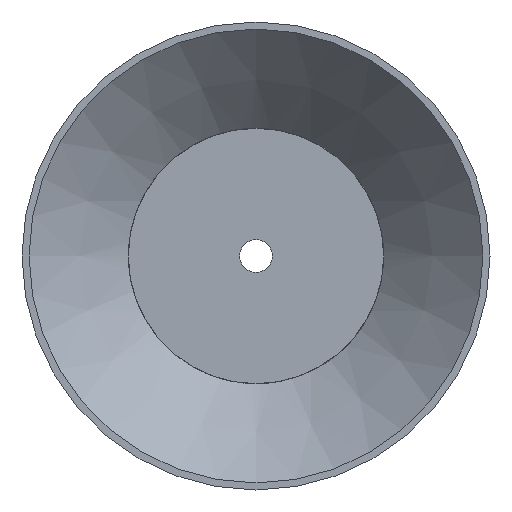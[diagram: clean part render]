
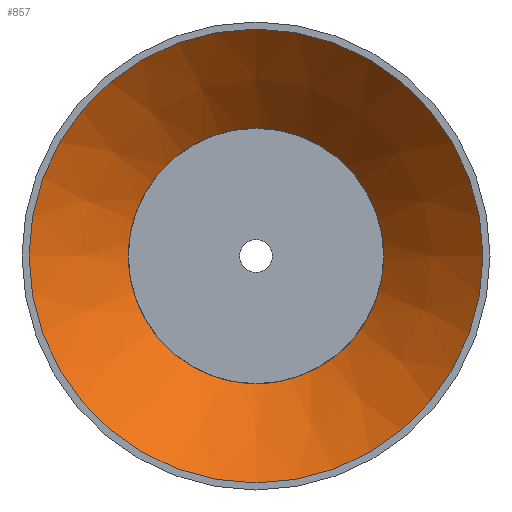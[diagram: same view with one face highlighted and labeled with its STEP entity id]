
A CAD part, front view. The second image highlights one B-rep face of the part: STEP entity #857.
In plain terms, the highlighted conical face has half-angle 45.227 degrees and reference radius 31.679 mm.
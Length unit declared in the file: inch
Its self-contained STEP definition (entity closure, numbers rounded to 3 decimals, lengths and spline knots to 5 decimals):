
#45=CONICAL_SURFACE('',#924,1.24722,0.789);
#54=LINE('',#1304,#84);
#84=VECTOR('',#1017,1.24722);
#116=(
BOUNDED_CURVE()
B_SPLINE_CURVE(2,(#1307,#1308,#1309),.UNSPECIFIED.,.F.,.F.)
B_SPLINE_CURVE_WITH_KNOTS((3,3),(0.,0.0225),.UNSPECIFIED.)
CURVE()
GEOMETRIC_REPRESENTATION_ITEM()
RATIONAL_B_SPLINE_CURVE((1.,1.,1.))
REPRESENTATION_ITEM('')
);
#117=(
BOUNDED_CURVE()
B_SPLINE_CURVE(2,(#1311,#1312,#1313),.UNSPECIFIED.,.F.,.F.)
B_SPLINE_CURVE_WITH_KNOTS((3,3),(0.8627,0.8852),
 .UNSPECIFIED.)
CURVE()
GEOMETRIC_REPRESENTATION_ITEM()
RATIONAL_B_SPLINE_CURVE((1.,1.,1.))
REPRESENTATION_ITEM('')
);
#118=(
BOUNDED_CURVE()
B_SPLINE_CURVE(2,(#1316,#1317,#1318),.UNSPECIFIED.,.F.,.F.)
B_SPLINE_CURVE_WITH_KNOTS((3,3),(0.,0.0225),.UNSPECIFIED.)
CURVE()
GEOMETRIC_REPRESENTATION_ITEM()
RATIONAL_B_SPLINE_CURVE((1.,1.,1.))
REPRESENTATION_ITEM('')
);
#119=(
BOUNDED_CURVE()
B_SPLINE_CURVE(2,(#1320,#1321,#1322),.UNSPECIFIED.,.F.,.F.)
B_SPLINE_CURVE_WITH_KNOTS((3,3),(0.86268,0.88518),
 .UNSPECIFIED.)
CURVE()
GEOMETRIC_REPRESENTATION_ITEM()
RATIONAL_B_SPLINE_CURVE((1.,1.,1.))
REPRESENTATION_ITEM('')
);
#120=(
BOUNDED_CURVE()
B_SPLINE_CURVE(2,(#1325,#1326,#1327),.UNSPECIFIED.,.F.,.F.)
B_SPLINE_CURVE_WITH_KNOTS((3,3),(0.,0.0225),.UNSPECIFIED.)
CURVE()
GEOMETRIC_REPRESENTATION_ITEM()
RATIONAL_B_SPLINE_CURVE((1.,1.,1.))
REPRESENTATION_ITEM('')
);
#121=(
BOUNDED_CURVE()
B_SPLINE_CURVE(2,(#1329,#1330,#1331),.UNSPECIFIED.,.F.,.F.)
B_SPLINE_CURVE_WITH_KNOTS((3,3),(0.86263,0.88513),
 .UNSPECIFIED.)
CURVE()
GEOMETRIC_REPRESENTATION_ITEM()
RATIONAL_B_SPLINE_CURVE((1.,1.,1.))
REPRESENTATION_ITEM('')
);
#122=(
BOUNDED_CURVE()
B_SPLINE_CURVE(2,(#1335,#1336,#1337),.UNSPECIFIED.,.F.,.F.)
B_SPLINE_CURVE_WITH_KNOTS((3,3),(0.,0.0225),.UNSPECIFIED.)
CURVE()
GEOMETRIC_REPRESENTATION_ITEM()
RATIONAL_B_SPLINE_CURVE((1.,1.,1.))
REPRESENTATION_ITEM('')
);
#123=(
BOUNDED_CURVE()
B_SPLINE_CURVE(2,(#1341,#1342,#1343),.UNSPECIFIED.,.F.,.F.)
B_SPLINE_CURVE_WITH_KNOTS((3,3),(0.86258,0.88508),
 .UNSPECIFIED.)
CURVE()
GEOMETRIC_REPRESENTATION_ITEM()
RATIONAL_B_SPLINE_CURVE((1.,1.,1.))
REPRESENTATION_ITEM('')
);
#203=FACE_OUTER_BOUND('',#243,.T.);
#243=EDGE_LOOP('',(#606,#607,#608,#609,#610,#611,#612,#613,#614,#615,#616,
#617,#618,#619,#620,#621,#622,#623,#624,#625,#626));
#291=CIRCLE('',#919,0.89444);
#292=CIRCLE('',#921,0.89444);
#293=CIRCLE('',#923,0.89444);
#294=CIRCLE('',#925,1.6);
#295=CIRCLE('',#926,0.9);
#296=CIRCLE('',#927,0.9);
#297=CIRCLE('',#928,0.9);
#298=CIRCLE('',#929,0.9);
#299=CIRCLE('',#930,0.89444);
#300=CIRCLE('',#931,0.9);
#301=CIRCLE('',#932,1.6);
#338=VERTEX_POINT('',#1282);
#339=VERTEX_POINT('',#1284);
#340=VERTEX_POINT('',#1288);
#341=VERTEX_POINT('',#1290);
#342=VERTEX_POINT('',#1294);
#343=VERTEX_POINT('',#1296);
#344=VERTEX_POINT('',#1300);
#345=VERTEX_POINT('',#1301);
#346=VERTEX_POINT('',#1303);
#347=VERTEX_POINT('',#1305);
#348=VERTEX_POINT('',#1310);
#349=VERTEX_POINT('',#1314);
#350=VERTEX_POINT('',#1319);
#351=VERTEX_POINT('',#1323);
#352=VERTEX_POINT('',#1328);
#353=VERTEX_POINT('',#1332);
#354=VERTEX_POINT('',#1334);
#355=VERTEX_POINT('',#1338);
#356=VERTEX_POINT('',#1340);
#443=EDGE_CURVE('',#339,#338,#291,.T.);
#446=EDGE_CURVE('',#341,#340,#292,.T.);
#448=EDGE_CURVE('',#342,#343,#293,.T.);
#450=EDGE_CURVE('',#344,#345,#294,.T.);
#451=EDGE_CURVE('',#345,#346,#54,.T.);
#452=EDGE_CURVE('',#347,#346,#295,.T.);
#453=EDGE_CURVE('',#340,#347,#116,.T.);
#454=EDGE_CURVE('',#348,#341,#117,.T.);
#455=EDGE_CURVE('',#349,#348,#296,.T.);
#456=EDGE_CURVE('',#338,#349,#118,.T.);
#457=EDGE_CURVE('',#350,#339,#119,.T.);
#458=EDGE_CURVE('',#351,#350,#297,.T.);
#459=EDGE_CURVE('',#343,#351,#120,.T.);
#460=EDGE_CURVE('',#352,#342,#121,.T.);
#461=EDGE_CURVE('',#353,#352,#298,.T.);
#462=EDGE_CURVE('',#354,#353,#122,.T.);
#463=EDGE_CURVE('',#355,#354,#299,.T.);
#464=EDGE_CURVE('',#356,#355,#123,.T.);
#465=EDGE_CURVE('',#346,#356,#300,.T.);
#466=EDGE_CURVE('',#345,#344,#301,.T.);
#606=ORIENTED_EDGE('',*,*,#450,.T.);
#607=ORIENTED_EDGE('',*,*,#451,.T.);
#608=ORIENTED_EDGE('',*,*,#452,.F.);
#609=ORIENTED_EDGE('',*,*,#453,.F.);
#610=ORIENTED_EDGE('',*,*,#446,.F.);
#611=ORIENTED_EDGE('',*,*,#454,.F.);
#612=ORIENTED_EDGE('',*,*,#455,.F.);
#613=ORIENTED_EDGE('',*,*,#456,.F.);
#614=ORIENTED_EDGE('',*,*,#443,.F.);
#615=ORIENTED_EDGE('',*,*,#457,.F.);
#616=ORIENTED_EDGE('',*,*,#458,.F.);
#617=ORIENTED_EDGE('',*,*,#459,.F.);
#618=ORIENTED_EDGE('',*,*,#448,.F.);
#619=ORIENTED_EDGE('',*,*,#460,.F.);
#620=ORIENTED_EDGE('',*,*,#461,.F.);
#621=ORIENTED_EDGE('',*,*,#462,.F.);
#622=ORIENTED_EDGE('',*,*,#463,.F.);
#623=ORIENTED_EDGE('',*,*,#464,.F.);
#624=ORIENTED_EDGE('',*,*,#465,.F.);
#625=ORIENTED_EDGE('',*,*,#451,.F.);
#626=ORIENTED_EDGE('',*,*,#466,.T.);
#857=ADVANCED_FACE('',(#203),#45,.F.);
#919=AXIS2_PLACEMENT_3D('',#1286,#999,#1000);
#921=AXIS2_PLACEMENT_3D('',#1292,#1005,#1006);
#923=AXIS2_PLACEMENT_3D('',#1297,#1010,#1011);
#924=AXIS2_PLACEMENT_3D('',#1299,#1013,#1014);
#925=AXIS2_PLACEMENT_3D('',#1302,#1015,#1016);
#926=AXIS2_PLACEMENT_3D('',#1306,#1018,#1019);
#927=AXIS2_PLACEMENT_3D('',#1315,#1020,#1021);
#928=AXIS2_PLACEMENT_3D('',#1324,#1022,#1023);
#929=AXIS2_PLACEMENT_3D('',#1333,#1024,#1025);
#930=AXIS2_PLACEMENT_3D('',#1339,#1026,#1027);
#931=AXIS2_PLACEMENT_3D('',#1344,#1028,#1029);
#932=AXIS2_PLACEMENT_3D('',#1345,#1030,#1031);
#999=DIRECTION('center_axis',(0.,-1.,0.));
#1000=DIRECTION('ref_axis',(1.,0.,0.));
#1005=DIRECTION('center_axis',(0.,-1.,0.));
#1006=DIRECTION('ref_axis',(1.,0.,0.));
#1010=DIRECTION('center_axis',(0.,-1.,0.));
#1011=DIRECTION('ref_axis',(1.,0.,0.));
#1013=DIRECTION('center_axis',(0.,-1.,0.));
#1014=DIRECTION('ref_axis',(1.,0.,0.));
#1015=DIRECTION('center_axis',(0.,-1.,0.));
#1016=DIRECTION('ref_axis',(1.,0.,0.));
#1017=DIRECTION('',(0.71,0.704,0.));
#1018=DIRECTION('center_axis',(0.,-1.,0.));
#1019=DIRECTION('ref_axis',(1.,0.,0.));
#1020=DIRECTION('center_axis',(0.,-1.,0.));
#1021=DIRECTION('ref_axis',(1.,0.,0.));
#1022=DIRECTION('center_axis',(0.,-1.,0.));
#1023=DIRECTION('ref_axis',(1.,0.,0.));
#1024=DIRECTION('center_axis',(0.,-1.,0.));
#1025=DIRECTION('ref_axis',(1.,0.,0.));
#1026=DIRECTION('center_axis',(0.,-1.,0.));
#1027=DIRECTION('ref_axis',(1.,0.,0.));
#1028=DIRECTION('center_axis',(0.,-1.,0.));
#1029=DIRECTION('ref_axis',(1.,0.,0.));
#1030=DIRECTION('center_axis',(0.,-1.,0.));
#1031=DIRECTION('ref_axis',(1.,0.,0.));
#1282=CARTESIAN_POINT('',(0.09988,0.7,0.88884));
#1284=CARTESIAN_POINT('',(0.88884,0.7,0.09991));
#1286=CARTESIAN_POINT('Origin',(0.,0.7,0.));
#1288=CARTESIAN_POINT('',(-0.88885,0.7,0.09984));
#1290=CARTESIAN_POINT('',(-0.09989,0.7,0.88884));
#1292=CARTESIAN_POINT('Origin',(0.,0.7,0.));
#1294=CARTESIAN_POINT('',(0.09995,0.7,-0.88883));
#1296=CARTESIAN_POINT('',(0.88879,0.7,-0.10031));
#1297=CARTESIAN_POINT('Origin',(0.,0.7,0.));
#1299=CARTESIAN_POINT('Origin',(0.,0.35,
0.));
#1300=CARTESIAN_POINT('',(1.6,0.,0.));
#1301=CARTESIAN_POINT('',(-1.6,0.,0.));
#1302=CARTESIAN_POINT('Origin',(0.,0.,
0.));
#1303=CARTESIAN_POINT('',(-0.9,0.69448,0.));
#1304=CARTESIAN_POINT('',(-1.24722,0.35,0.));
#1305=CARTESIAN_POINT('',(-0.89445,0.69448,0.09984));
#1306=CARTESIAN_POINT('Origin',(0.,0.69448,0.));
#1307=CARTESIAN_POINT('Ctrl Pts',(-0.88885,0.7,
0.09984));
#1308=CARTESIAN_POINT('Ctrl Pts',(-0.89164,0.69725,0.09984));
#1309=CARTESIAN_POINT('Ctrl Pts',(-0.89445,0.69448,
0.09984));
#1310=CARTESIAN_POINT('',(-0.09989,0.69448,0.89444));
#1311=CARTESIAN_POINT('Ctrl Pts',(-0.09989,0.69448,
0.89444));
#1312=CARTESIAN_POINT('Ctrl Pts',(-0.09989,0.69725,
0.89163));
#1313=CARTESIAN_POINT('Ctrl Pts',(-0.09989,0.7,
0.88884));
#1314=CARTESIAN_POINT('',(0.09988,0.69448,0.89444));
#1315=CARTESIAN_POINT('Origin',(0.,0.69448,0.));
#1316=CARTESIAN_POINT('Ctrl Pts',(0.09988,0.7,
0.88884));
#1317=CARTESIAN_POINT('Ctrl Pts',(0.09988,0.69725,
0.89163));
#1318=CARTESIAN_POINT('Ctrl Pts',(0.09988,0.69448,
0.89444));
#1319=CARTESIAN_POINT('',(0.89444,0.69448,0.09991));
#1320=CARTESIAN_POINT('Ctrl Pts',(0.89444,0.69448,0.09991));
#1321=CARTESIAN_POINT('Ctrl Pts',(0.89163,0.69725,0.09991));
#1322=CARTESIAN_POINT('Ctrl Pts',(0.88884,0.7,0.09991));
#1323=CARTESIAN_POINT('',(0.89439,0.69448,-0.10032));
#1324=CARTESIAN_POINT('Origin',(0.,0.69448,0.));
#1325=CARTESIAN_POINT('Ctrl Pts',(0.88879,0.7,-0.10031));
#1326=CARTESIAN_POINT('Ctrl Pts',(0.89158,0.69725,-0.10032));
#1327=CARTESIAN_POINT('Ctrl Pts',(0.89439,0.69448,-0.10032));
#1328=CARTESIAN_POINT('',(0.09995,0.69448,-0.89443));
#1329=CARTESIAN_POINT('Ctrl Pts',(0.09995,0.69448,
-0.89443));
#1330=CARTESIAN_POINT('Ctrl Pts',(0.09995,0.69725,-0.89162));
#1331=CARTESIAN_POINT('Ctrl Pts',(0.09995,0.7,
-0.88883));
#1332=CARTESIAN_POINT('',(-0.09955,0.69448,-0.89448));
#1333=CARTESIAN_POINT('Origin',(0.,0.69448,0.));
#1334=CARTESIAN_POINT('',(-0.09956,0.7,-0.88888));
#1335=CARTESIAN_POINT('Ctrl Pts',(-0.09956,0.7,
-0.88888));
#1336=CARTESIAN_POINT('Ctrl Pts',(-0.09956,0.69725,
-0.89167));
#1337=CARTESIAN_POINT('Ctrl Pts',(-0.09955,0.69448,
-0.89448));
#1338=CARTESIAN_POINT('',(-0.88883,0.7,-0.1));
#1339=CARTESIAN_POINT('Origin',(0.,0.7,0.));
#1340=CARTESIAN_POINT('',(-0.89443,0.69448,-0.1));
#1341=CARTESIAN_POINT('Ctrl Pts',(-0.89443,0.69448,
-0.1));
#1342=CARTESIAN_POINT('Ctrl Pts',(-0.89162,0.69725,
-0.1));
#1343=CARTESIAN_POINT('Ctrl Pts',(-0.88883,0.7,
-0.1));
#1344=CARTESIAN_POINT('Origin',(0.,0.69448,0.));
#1345=CARTESIAN_POINT('Origin',(0.,0.,
0.));
